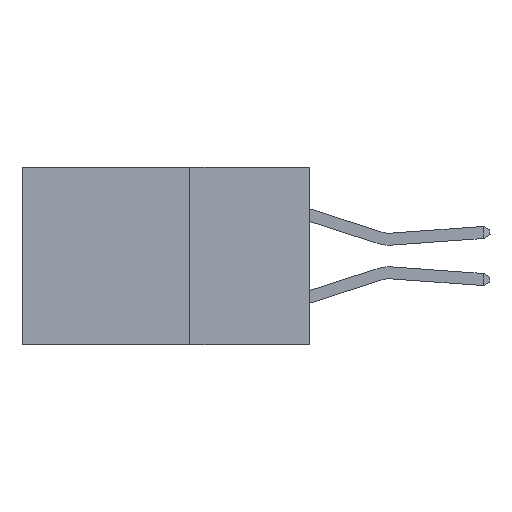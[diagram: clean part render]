
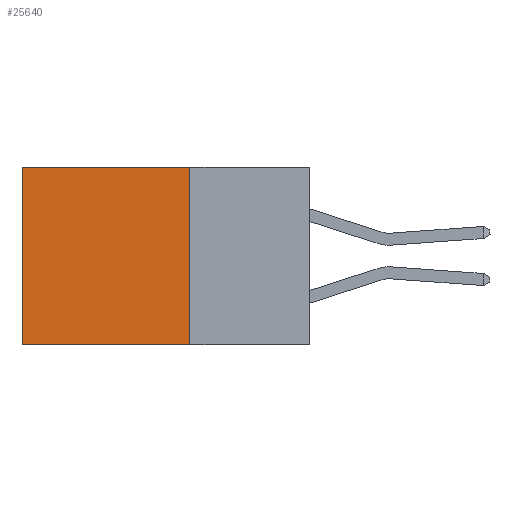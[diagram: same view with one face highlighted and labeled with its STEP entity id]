
A CAD part, left-side view. The second image highlights one B-rep face of the part: STEP entity #25640.
In plain terms, the highlighted planar face has unit normal (-1, 0, 0).
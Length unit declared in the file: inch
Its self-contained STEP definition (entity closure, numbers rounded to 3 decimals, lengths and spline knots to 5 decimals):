
#1488 = DIRECTION ( 'NONE',  ( 1., 0., 0. ) ) ;
#1511 = EDGE_CURVE ( 'NONE', #20219, #4498, #26150, .T. ) ;
#3022 = EDGE_LOOP ( 'NONE', ( #7199, #15271, #22350, #22978 ) ) ;
#3381 = LINE ( 'NONE', #7103, #32340 ) ;
#3814 = PLANE ( 'NONE',  #18396 ) ;
#4498 = VERTEX_POINT ( 'NONE', #29444 ) ;
#5202 = CARTESIAN_POINT ( 'NONE',  ( 0.298, 0.6, 0. ) ) ;
#6798 = EDGE_CURVE ( 'NONE', #32049, #11785, #15838, .T. ) ;
#7103 = CARTESIAN_POINT ( 'NONE',  ( 0.298, 0.25, 0. ) ) ;
#7199 = ORIENTED_EDGE ( 'NONE', *, *, #1511, .T. ) ;
#8087 = VECTOR ( 'NONE', #11664, 39.37008 ) ;
#8129 = LINE ( 'NONE', #18368, #23771 ) ;
#8376 = CARTESIAN_POINT ( 'NONE',  ( 0.298, 0.25, 0. ) ) ;
#10475 = EDGE_CURVE ( 'NONE', #32049, #20219, #3381, .T. ) ;
#11664 = DIRECTION ( 'NONE',  ( 0., 0., -1. ) ) ;
#11785 = VERTEX_POINT ( 'NONE', #11795 ) ;
#11795 = CARTESIAN_POINT ( 'NONE',  ( 0.298, 0.25, -0.37 ) ) ;
#13332 = CARTESIAN_POINT ( 'NONE',  ( 0.298, 0.25, 0. ) ) ;
#15271 = ORIENTED_EDGE ( 'NONE', *, *, #28827, .F. ) ;
#15838 = LINE ( 'NONE', #13332, #28730 ) ;
#16298 = DIRECTION ( 'NONE',  ( 0., 0., -1. ) ) ;
#16792 = CARTESIAN_POINT ( 'NONE',  ( 0.298, 0.6, 0. ) ) ;
#18004 = FACE_OUTER_BOUND ( 'NONE', #3022, .T. ) ;
#18368 = CARTESIAN_POINT ( 'NONE',  ( 0.298, 0.25, -0.37 ) ) ;
#18396 = AXIS2_PLACEMENT_3D ( 'NONE', #27292, #1488, #32250 ) ;
#20219 = VERTEX_POINT ( 'NONE', #5202 ) ;
#21290 = DIRECTION ( 'NONE',  ( 0., 1., 0. ) ) ;
#22350 = ORIENTED_EDGE ( 'NONE', *, *, #6798, .F. ) ;
#22978 = ORIENTED_EDGE ( 'NONE', *, *, #10475, .T. ) ;
#23771 = VECTOR ( 'NONE', #21290, 39.37008 ) ;
#25640 = ADVANCED_FACE ( 'NONE', ( #18004 ), #3814, .F. ) ;
#25844 = DIRECTION ( 'NONE',  ( 0., 1., 0. ) ) ;
#26150 = LINE ( 'NONE', #16792, #8087 ) ;
#27292 = CARTESIAN_POINT ( 'NONE',  ( 0.298, 0.25, 0. ) ) ;
#28730 = VECTOR ( 'NONE', #16298, 39.37008 ) ;
#28827 = EDGE_CURVE ( 'NONE', #11785, #4498, #8129, .T. ) ;
#29444 = CARTESIAN_POINT ( 'NONE',  ( 0.298, 0.6, -0.37 ) ) ;
#32049 = VERTEX_POINT ( 'NONE', #8376 ) ;
#32250 = DIRECTION ( 'NONE',  ( 0., 0., -1. ) ) ;
#32340 = VECTOR ( 'NONE', #25844, 39.37008 ) ;
